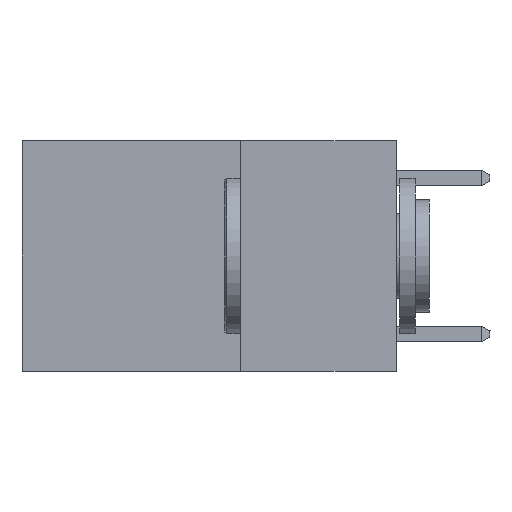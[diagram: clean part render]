
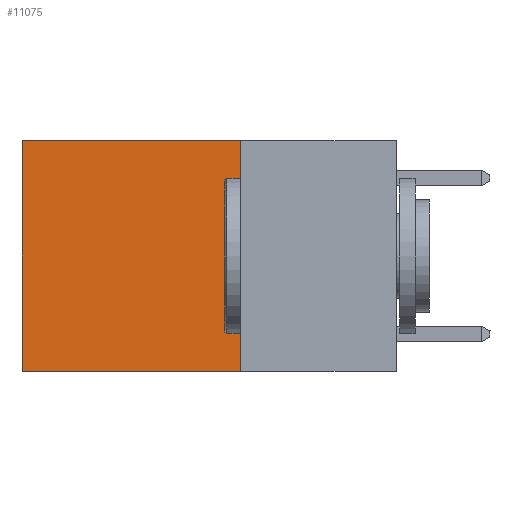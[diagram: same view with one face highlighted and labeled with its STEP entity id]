
A CAD part, left-side view. The second image highlights one B-rep face of the part: STEP entity #11075.
In plain terms, the highlighted planar face has unit normal (-1, 0, 0).
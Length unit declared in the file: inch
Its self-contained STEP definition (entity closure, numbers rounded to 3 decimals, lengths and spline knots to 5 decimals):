
#271 = EDGE_CURVE ( 'NONE', #5900, #6471, #2832, .T. ) ;
#980 = DIRECTION ( 'NONE',  ( 0., 1., 0. ) ) ;
#1312 = VECTOR ( 'NONE', #4817, 39.37008 ) ;
#1796 = ORIENTED_EDGE ( 'NONE', *, *, #11621, .F. ) ;
#1972 = VERTEX_POINT ( 'NONE', #4834 ) ;
#2299 = DIRECTION ( 'NONE',  ( 0., 0., -1. ) ) ;
#2339 = ORIENTED_EDGE ( 'NONE', *, *, #2894, .T. ) ;
#2613 = VECTOR ( 'NONE', #2299, 39.37008 ) ;
#2738 = CARTESIAN_POINT ( 'NONE',  ( 0.2625, 0.6, 0. ) ) ;
#2832 = LINE ( 'NONE', #4027, #6747 ) ;
#2894 = EDGE_CURVE ( 'NONE', #6471, #1972, #5250, .T. ) ;
#3446 = LINE ( 'NONE', #8563, #1312 ) ;
#3827 = LINE ( 'NONE', #9960, #2613 ) ;
#4027 = CARTESIAN_POINT ( 'NONE',  ( 0.2625, 0.25, 0. ) ) ;
#4501 = PLANE ( 'NONE',  #9835 ) ;
#4817 = DIRECTION ( 'NONE',  ( 0., 1., 0. ) ) ;
#4834 = CARTESIAN_POINT ( 'NONE',  ( 0.2625, 0.6, -0.37 ) ) ;
#5250 = LINE ( 'NONE', #2738, #11029 ) ;
#5900 = VERTEX_POINT ( 'NONE', #11891 ) ;
#6140 = CARTESIAN_POINT ( 'NONE',  ( 0.2625, 0.6, 0. ) ) ;
#6471 = VERTEX_POINT ( 'NONE', #6140 ) ;
#6505 = EDGE_CURVE ( 'NONE', #5900, #7175, #3827, .T. ) ;
#6747 = VECTOR ( 'NONE', #980, 39.37008 ) ;
#7175 = VERTEX_POINT ( 'NONE', #9841 ) ;
#7473 = CARTESIAN_POINT ( 'NONE',  ( 0.2625, 0.25, 0. ) ) ;
#7856 = EDGE_LOOP ( 'NONE', ( #2339, #1796, #9106, #8664 ) ) ;
#8563 = CARTESIAN_POINT ( 'NONE',  ( 0.2625, 0.25, -0.37 ) ) ;
#8664 = ORIENTED_EDGE ( 'NONE', *, *, #271, .T. ) ;
#9106 = ORIENTED_EDGE ( 'NONE', *, *, #6505, .F. ) ;
#9434 = DIRECTION ( 'NONE',  ( 0., 0., -1. ) ) ;
#9515 = DIRECTION ( 'NONE',  ( 0., 0., -1. ) ) ;
#9835 = AXIS2_PLACEMENT_3D ( 'NONE', #7473, #12276, #9434 ) ;
#9841 = CARTESIAN_POINT ( 'NONE',  ( 0.2625, 0.25, -0.37 ) ) ;
#9960 = CARTESIAN_POINT ( 'NONE',  ( 0.2625, 0.25, 0. ) ) ;
#11029 = VECTOR ( 'NONE', #9515, 39.37008 ) ;
#11075 = ADVANCED_FACE ( 'NONE', ( #11217 ), #4501, .F. ) ;
#11217 = FACE_OUTER_BOUND ( 'NONE', #7856, .T. ) ;
#11621 = EDGE_CURVE ( 'NONE', #7175, #1972, #3446, .T. ) ;
#11891 = CARTESIAN_POINT ( 'NONE',  ( 0.2625, 0.25, 0. ) ) ;
#12276 = DIRECTION ( 'NONE',  ( 1., 0., 0. ) ) ;
